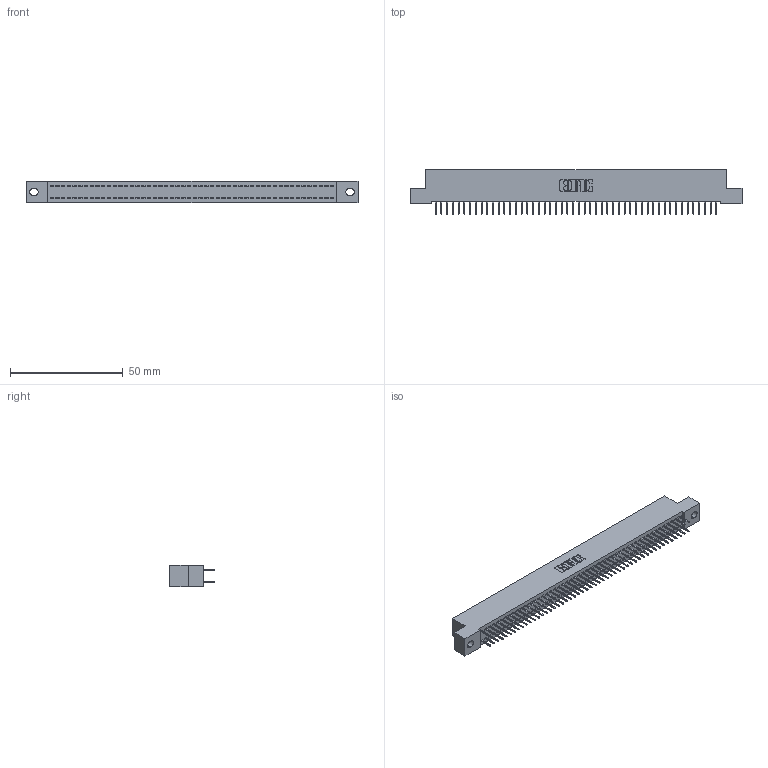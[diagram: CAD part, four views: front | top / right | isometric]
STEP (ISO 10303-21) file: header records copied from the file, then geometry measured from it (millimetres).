
FILE_DESCRIPTION (( 'STEP AP203' ), '1' );
FILE_NAME ('392-100-524-202.STEP', '2019-10-09T20:48:05', ( '' ), ( '' ), 'SwSTEP 2.0', 'SolidWorks 2016', '' );
FILE_SCHEMA (( 'CONFIG_CONTROL_DESIGN' ));
Length unit declared in the file: inch
Products named in the file (3): 342 Part_.128 Slot; 345-292-001_345-293-124; 392-100-524-202
Assembly tree (101 placements, depth 2):
  392-100-524-202
    342 Part_.128 Slot
    345-292-001_345-293-124  x100
Bounding box: 147.32 x 19.69 x 9.4 mm (x, y, z)
Volume: 13071.1 mm3; surface area: 20839.4 mm2
Topology: 101 solids, 101 shells, 5714 faces, 16211 edges, 10406 vertices
Faces by surface type: plane 4270, cylinder 1444
Entity records: 31209 total; most frequent: CARTESIAN_POINT 5162, ORIENTED_EDGE 5098, DIRECTION 4397, EDGE_CURVE 2549, VECTOR 2425, LINE 2425, VERTEX_POINT 1694, AXIS2_PLACEMENT_3D 986
